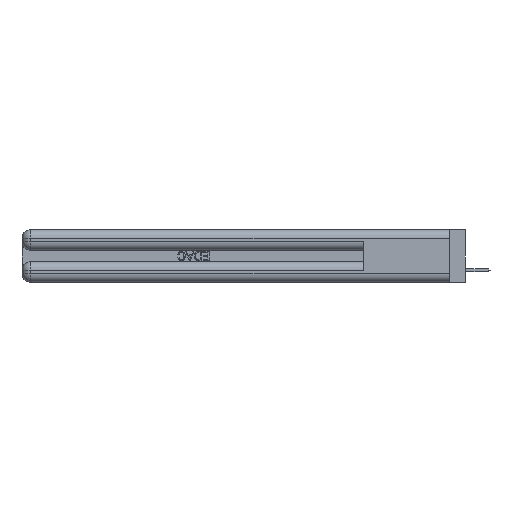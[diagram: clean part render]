
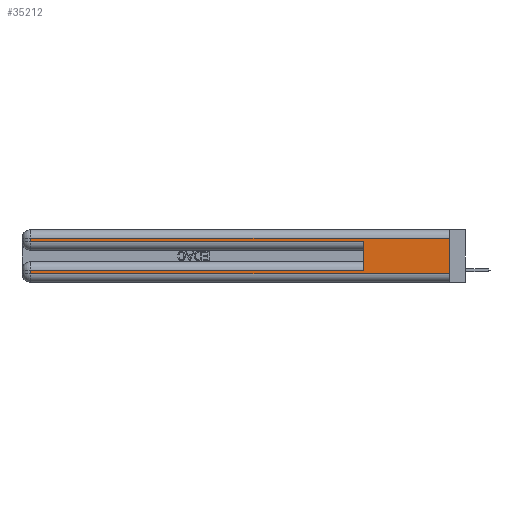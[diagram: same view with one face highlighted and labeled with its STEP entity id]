
A CAD part, left-side view. The second image highlights one B-rep face of the part: STEP entity #35212.
In plain terms, the highlighted planar face has unit normal (-1, 0, 0).
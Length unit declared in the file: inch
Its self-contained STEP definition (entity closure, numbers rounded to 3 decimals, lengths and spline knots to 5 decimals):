
#257 = CARTESIAN_POINT ( 'NONE',  ( 0., 0., 0.31 ) ) ;
#728 = VECTOR ( 'NONE', #2643, 39.37008 ) ;
#880 = DIRECTION ( 'NONE',  ( 0., 0., 1. ) ) ;
#1313 = EDGE_LOOP ( 'NONE', ( #33162, #11614, #15242, #28318, #9647, #5672, #21329, #16921 ) ) ;
#1606 = VECTOR ( 'NONE', #24392, 39.37008 ) ;
#1928 = LINE ( 'NONE', #37765, #7379 ) ;
#2627 = VERTEX_POINT ( 'NONE', #7708 ) ;
#2643 = DIRECTION ( 'NONE',  ( 0., 0., -1. ) ) ;
#2847 = VERTEX_POINT ( 'NONE', #35088 ) ;
#3873 = CARTESIAN_POINT ( 'NONE',  ( 0., 2.94, 0.31 ) ) ;
#5116 = VECTOR ( 'NONE', #20316, 39.37008 ) ;
#5672 = ORIENTED_EDGE ( 'NONE', *, *, #31535, .T. ) ;
#6071 = CARTESIAN_POINT ( 'NONE',  ( 0., 2.94, 0.37 ) ) ;
#6203 = CARTESIAN_POINT ( 'NONE',  ( 0., 0.6, 0.145 ) ) ;
#7374 = EDGE_CURVE ( 'NONE', #20634, #25696, #17524, .T. ) ;
#7379 = VECTOR ( 'NONE', #12021, 39.37008 ) ;
#7517 = CARTESIAN_POINT ( 'NONE',  ( 0., 0., 0.31 ) ) ;
#7708 = CARTESIAN_POINT ( 'NONE',  ( 0., 0.6, 0.285 ) ) ;
#8094 = VERTEX_POINT ( 'NONE', #9327 ) ;
#8642 = AXIS2_PLACEMENT_3D ( 'NONE', #10064, #16445, #13707 ) ;
#8684 = CARTESIAN_POINT ( 'NONE',  ( 0., 2.94, 0.085 ) ) ;
#9327 = CARTESIAN_POINT ( 'NONE',  ( 0., 2.94, 0.285 ) ) ;
#9647 = ORIENTED_EDGE ( 'NONE', *, *, #14271, .F. ) ;
#10064 = CARTESIAN_POINT ( 'NONE',  ( 0., 0., 0.37 ) ) ;
#10126 = EDGE_CURVE ( 'NONE', #40948, #11900, #10678, .T. ) ;
#10678 = LINE ( 'NONE', #37531, #728 ) ;
#11614 = ORIENTED_EDGE ( 'NONE', *, *, #7374, .T. ) ;
#11900 = VERTEX_POINT ( 'NONE', #22964 ) ;
#12021 = DIRECTION ( 'NONE',  ( 0., 1., 0. ) ) ;
#12351 = EDGE_CURVE ( 'NONE', #11900, #2847, #24591, .T. ) ;
#13281 = PLANE ( 'NONE',  #8642 ) ;
#13491 = LINE ( 'NONE', #6203, #30031 ) ;
#13707 = DIRECTION ( 'NONE',  ( 0., 0., -1. ) ) ;
#14271 = EDGE_CURVE ( 'NONE', #33458, #2627, #13491, .T. ) ;
#15242 = ORIENTED_EDGE ( 'NONE', *, *, #23500, .T. ) ;
#15381 = EDGE_CURVE ( 'NONE', #20634, #2847, #18894, .T. ) ;
#15799 = DIRECTION ( 'NONE',  ( 0., 0., -1. ) ) ;
#16066 = CARTESIAN_POINT ( 'NONE',  ( 0., 0., 0.37 ) ) ;
#16445 = DIRECTION ( 'NONE',  ( 1., 0., 0. ) ) ;
#16921 = ORIENTED_EDGE ( 'NONE', *, *, #12351, .T. ) ;
#16980 = LINE ( 'NONE', #6071, #19978 ) ;
#17168 = CARTESIAN_POINT ( 'NONE',  ( 0., 0., 0.285 ) ) ;
#17440 = LINE ( 'NONE', #17168, #23496 ) ;
#17524 = LINE ( 'NONE', #7517, #5116 ) ;
#17899 = CARTESIAN_POINT ( 'NONE',  ( 0., 0., 0.06 ) ) ;
#18894 = LINE ( 'NONE', #16066, #36934 ) ;
#19978 = VECTOR ( 'NONE', #15799, 39.37008 ) ;
#20316 = DIRECTION ( 'NONE',  ( 0., 1., 0. ) ) ;
#20634 = VERTEX_POINT ( 'NONE', #257 ) ;
#21329 = ORIENTED_EDGE ( 'NONE', *, *, #10126, .T. ) ;
#22964 = CARTESIAN_POINT ( 'NONE',  ( 0., 2.94, 0.06 ) ) ;
#23496 = VECTOR ( 'NONE', #36629, 39.37008 ) ;
#23500 = EDGE_CURVE ( 'NONE', #25696, #8094, #16980, .T. ) ;
#24260 = EDGE_CURVE ( 'NONE', #8094, #2627, #17440, .T. ) ;
#24392 = DIRECTION ( 'NONE',  ( 0., -1., 0. ) ) ;
#24591 = LINE ( 'NONE', #17899, #1606 ) ;
#25696 = VERTEX_POINT ( 'NONE', #3873 ) ;
#28318 = ORIENTED_EDGE ( 'NONE', *, *, #24260, .T. ) ;
#29820 = CARTESIAN_POINT ( 'NONE',  ( 0., 0.6, 0.085 ) ) ;
#30031 = VECTOR ( 'NONE', #880, 39.37008 ) ;
#31535 = EDGE_CURVE ( 'NONE', #33458, #40948, #1928, .T. ) ;
#33162 = ORIENTED_EDGE ( 'NONE', *, *, #15381, .F. ) ;
#33458 = VERTEX_POINT ( 'NONE', #29820 ) ;
#35088 = CARTESIAN_POINT ( 'NONE',  ( 0., 0., 0.06 ) ) ;
#35129 = DIRECTION ( 'NONE',  ( 0., 0., -1. ) ) ;
#35212 = ADVANCED_FACE ( 'NONE', ( #35723 ), #13281, .F. ) ;
#35723 = FACE_OUTER_BOUND ( 'NONE', #1313, .T. ) ;
#36629 = DIRECTION ( 'NONE',  ( 0., -1., 0. ) ) ;
#36934 = VECTOR ( 'NONE', #35129, 39.37008 ) ;
#37531 = CARTESIAN_POINT ( 'NONE',  ( 0., 2.94, 0.37 ) ) ;
#37765 = CARTESIAN_POINT ( 'NONE',  ( 0., 0., 0.085 ) ) ;
#40948 = VERTEX_POINT ( 'NONE', #8684 ) ;
